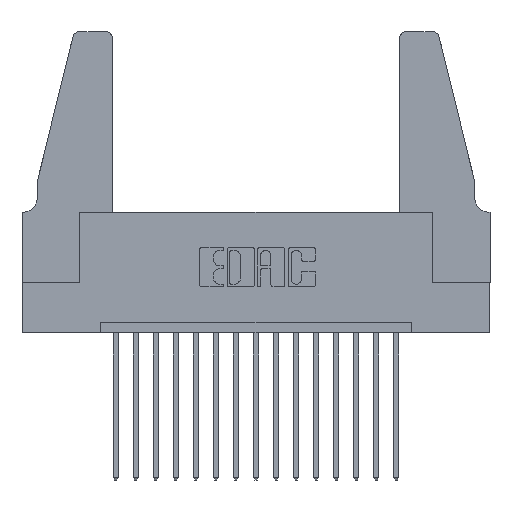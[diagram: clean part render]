
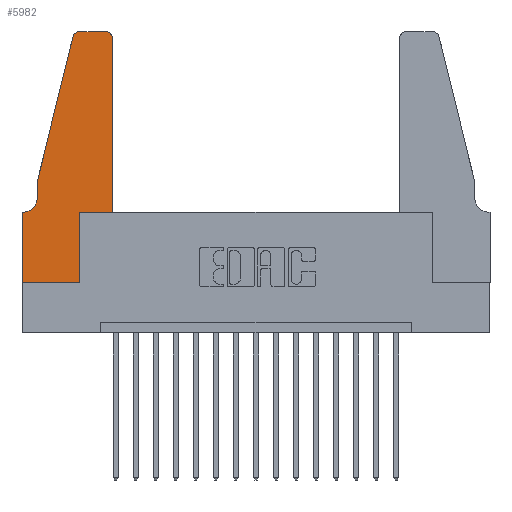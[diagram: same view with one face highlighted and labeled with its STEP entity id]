
A CAD part, top view. The second image highlights one B-rep face of the part: STEP entity #5982.
In plain terms, the highlighted planar face has unit normal (0, 0, 1).
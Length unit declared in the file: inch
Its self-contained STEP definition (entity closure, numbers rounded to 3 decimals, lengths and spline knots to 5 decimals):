
#80 = ORIENTED_EDGE ( 'NONE', *, *, #11843, .T. ) ;
#95 = EDGE_LOOP ( 'NONE', ( #4123, #4974, #15782, #13313, #5317, #12016, #80, #13211, #8680, #7948, #15334, #16169 ) ) ;
#119 = DIRECTION ( 'NONE',  ( 0., 1., 0. ) ) ;
#205 = CARTESIAN_POINT ( 'NONE',  ( 0.2865, 0., 0.37 ) ) ;
#444 = DIRECTION ( 'NONE',  ( 1., 0., 0. ) ) ;
#517 = CARTESIAN_POINT ( 'NONE',  ( 0.4205, 1.22, 0.37 ) ) ;
#1001 = CARTESIAN_POINT ( 'NONE',  ( 0.2605, 1.25, 0.37 ) ) ;
#1219 = DIRECTION ( 'NONE',  ( -1., 0., 0. ) ) ;
#1370 = CIRCLE ( 'NONE', #4798, 0.03 ) ;
#1647 = LINE ( 'NONE', #6966, #4972 ) ;
#2059 = DIRECTION ( 'NONE',  ( 0., 0., 1. ) ) ;
#2354 = EDGE_CURVE ( 'NONE', #16927, #14852, #16873, .T. ) ;
#2645 = VECTOR ( 'NONE', #1219, 39.37008 ) ;
#2704 = VERTEX_POINT ( 'NONE', #11078 ) ;
#2728 = EDGE_CURVE ( 'NONE', #2888, #5459, #16241, .T. ) ;
#2742 = CARTESIAN_POINT ( 'NONE',  ( 0.284, 1.25, 0.37 ) ) ;
#2888 = VERTEX_POINT ( 'NONE', #5062 ) ;
#3286 = DIRECTION ( 'NONE',  ( 0., -1., 0. ) ) ;
#3410 = DIRECTION ( 'NONE',  ( 1., 0., 0. ) ) ;
#3512 = VECTOR ( 'NONE', #9715, 39.37008 ) ;
#3623 = DIRECTION ( 'NONE',  ( -1., 0., 0. ) ) ;
#3637 = EDGE_CURVE ( 'NONE', #10289, #11066, #5955, .T. ) ;
#3641 = VERTEX_POINT ( 'NONE', #15367 ) ;
#3827 = EDGE_CURVE ( 'NONE', #11066, #12361, #14798, .T. ) ;
#3957 = EDGE_CURVE ( 'NONE', #13204, #10289, #14379, .T. ) ;
#4123 = ORIENTED_EDGE ( 'NONE', *, *, #3957, .T. ) ;
#4444 = VECTOR ( 'NONE', #3286, 39.37008 ) ;
#4655 = EDGE_CURVE ( 'NONE', #5459, #3641, #5757, .T. ) ;
#4660 = DIRECTION ( 'NONE',  ( 0., 0., -1. ) ) ;
#4706 = DIRECTION ( 'NONE',  ( 1., 0., 0. ) ) ;
#4798 = AXIS2_PLACEMENT_3D ( 'NONE', #517, #15092, #4706 ) ;
#4880 = VECTOR ( 'NONE', #444, 39.37008 ) ;
#4972 = VECTOR ( 'NONE', #119, 39.37008 ) ;
#4974 = ORIENTED_EDGE ( 'NONE', *, *, #3637, .T. ) ;
#5062 = CARTESIAN_POINT ( 'NONE',  ( 0.0755, 0.42, 0.37 ) ) ;
#5317 = ORIENTED_EDGE ( 'NONE', *, *, #2728, .T. ) ;
#5459 = VERTEX_POINT ( 'NONE', #8048 ) ;
#5757 = LINE ( 'NONE', #15692, #2645 ) ;
#5955 = CIRCLE ( 'NONE', #9656, 0.03 ) ;
#5982 = ADVANCED_FACE ( 'NONE', ( #12669 ), #7284, .T. ) ;
#6107 = DIRECTION ( 'NONE',  ( 0., 1., 0. ) ) ;
#6940 = CARTESIAN_POINT ( 'NONE',  ( 0.4505, 0.35, 0.37 ) ) ;
#6966 = CARTESIAN_POINT ( 'NONE',  ( 0.4505, 0.35, 0.37 ) ) ;
#6988 = CARTESIAN_POINT ( 'NONE',  ( 0.4505, 0.35, 0.37 ) ) ;
#7284 = PLANE ( 'NONE',  #10787 ) ;
#7885 = LINE ( 'NONE', #15230, #10770 ) ;
#7948 = ORIENTED_EDGE ( 'NONE', *, *, #17107, .T. ) ;
#8048 = CARTESIAN_POINT ( 'NONE',  ( 0.0055, 0.35, 0.37 ) ) ;
#8126 = CARTESIAN_POINT ( 'NONE',  ( 0.25487, 1.22718, 0.37 ) ) ;
#8447 = VERTEX_POINT ( 'NONE', #6940 ) ;
#8669 = DIRECTION ( 'NONE',  ( 0., -1., 0. ) ) ;
#8680 = ORIENTED_EDGE ( 'NONE', *, *, #2354, .T. ) ;
#8856 = CARTESIAN_POINT ( 'NONE',  ( 0.2865, 0.35, 0.37 ) ) ;
#9379 = LINE ( 'NONE', #6988, #4880 ) ;
#9570 = EDGE_CURVE ( 'NONE', #8447, #16305, #1647, .T. ) ;
#9656 = AXIS2_PLACEMENT_3D ( 'NONE', #16551, #2059, #3410 ) ;
#9715 = DIRECTION ( 'NONE',  ( -0.239, -0.971, 0. ) ) ;
#10289 = VERTEX_POINT ( 'NONE', #2742 ) ;
#10468 = EDGE_CURVE ( 'NONE', #16305, #13204, #1370, .T. ) ;
#10594 = CARTESIAN_POINT ( 'NONE',  ( 0., 0., 0.37 ) ) ;
#10731 = CARTESIAN_POINT ( 'NONE',  ( 0.4505, 1.22, 0.37 ) ) ;
#10770 = VECTOR ( 'NONE', #8669, 39.37008 ) ;
#10787 = AXIS2_PLACEMENT_3D ( 'NONE', #15101, #12460, #16522 ) ;
#11027 = CARTESIAN_POINT ( 'NONE',  ( 0.0055, 0.42, 0.37 ) ) ;
#11066 = VERTEX_POINT ( 'NONE', #8126 ) ;
#11078 = CARTESIAN_POINT ( 'NONE',  ( 0., 0., 0.37 ) ) ;
#11843 = EDGE_CURVE ( 'NONE', #3641, #2704, #15803, .T. ) ;
#12016 = ORIENTED_EDGE ( 'NONE', *, *, #4655, .T. ) ;
#12361 = VERTEX_POINT ( 'NONE', #14565 ) ;
#12408 = DIRECTION ( 'NONE',  ( -1., 0., 0. ) ) ;
#12410 = AXIS2_PLACEMENT_3D ( 'NONE', #11027, #4660, #12408 ) ;
#12460 = DIRECTION ( 'NONE',  ( 0., 0., 1. ) ) ;
#12486 = CARTESIAN_POINT ( 'NONE',  ( 0.0755, 0.5, 0.37 ) ) ;
#12669 = FACE_OUTER_BOUND ( 'NONE', #95, .T. ) ;
#13162 = LINE ( 'NONE', #10594, #13758 ) ;
#13204 = VERTEX_POINT ( 'NONE', #13822 ) ;
#13211 = ORIENTED_EDGE ( 'NONE', *, *, #15299, .T. ) ;
#13298 = EDGE_CURVE ( 'NONE', #12361, #2888, #7885, .T. ) ;
#13313 = ORIENTED_EDGE ( 'NONE', *, *, #13298, .T. ) ;
#13758 = VECTOR ( 'NONE', #15742, 39.37008 ) ;
#13822 = CARTESIAN_POINT ( 'NONE',  ( 0.4205, 1.25, 0.37 ) ) ;
#13954 = VECTOR ( 'NONE', #3623, 39.37008 ) ;
#14379 = LINE ( 'NONE', #1001, #13954 ) ;
#14565 = CARTESIAN_POINT ( 'NONE',  ( 0.0755, 0.5, 0.37 ) ) ;
#14798 = LINE ( 'NONE', #12486, #3512 ) ;
#14852 = VERTEX_POINT ( 'NONE', #14856 ) ;
#14856 = CARTESIAN_POINT ( 'NONE',  ( 0.2865, 0.35, 0.37 ) ) ;
#15092 = DIRECTION ( 'NONE',  ( 0., 0., 1. ) ) ;
#15101 = CARTESIAN_POINT ( 'NONE',  ( 0., 0.35, 0.37 ) ) ;
#15230 = CARTESIAN_POINT ( 'NONE',  ( 0.0755, 0.5, 0.37 ) ) ;
#15299 = EDGE_CURVE ( 'NONE', #2704, #16927, #13162, .T. ) ;
#15334 = ORIENTED_EDGE ( 'NONE', *, *, #9570, .T. ) ;
#15367 = CARTESIAN_POINT ( 'NONE',  ( 0., 0.35, 0.37 ) ) ;
#15692 = CARTESIAN_POINT ( 'NONE',  ( 0.0755, 0.35, 0.37 ) ) ;
#15742 = DIRECTION ( 'NONE',  ( 1., 0., 0. ) ) ;
#15782 = ORIENTED_EDGE ( 'NONE', *, *, #3827, .T. ) ;
#15803 = LINE ( 'NONE', #16431, #4444 ) ;
#16169 = ORIENTED_EDGE ( 'NONE', *, *, #10468, .T. ) ;
#16241 = CIRCLE ( 'NONE', #12410, 0.07 ) ;
#16259 = VECTOR ( 'NONE', #6107, 39.37008 ) ;
#16305 = VERTEX_POINT ( 'NONE', #10731 ) ;
#16431 = CARTESIAN_POINT ( 'NONE',  ( 0., 0., 0.37 ) ) ;
#16522 = DIRECTION ( 'NONE',  ( 1., 0., 0. ) ) ;
#16551 = CARTESIAN_POINT ( 'NONE',  ( 0.284, 1.22, 0.37 ) ) ;
#16873 = LINE ( 'NONE', #8856, #16259 ) ;
#16927 = VERTEX_POINT ( 'NONE', #205 ) ;
#17107 = EDGE_CURVE ( 'NONE', #14852, #8447, #9379, .T. ) ;
